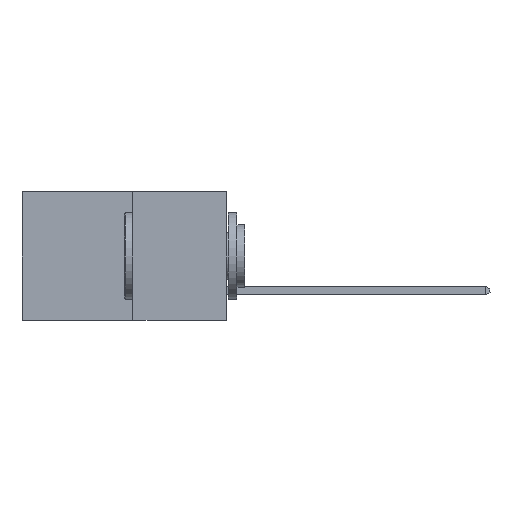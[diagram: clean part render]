
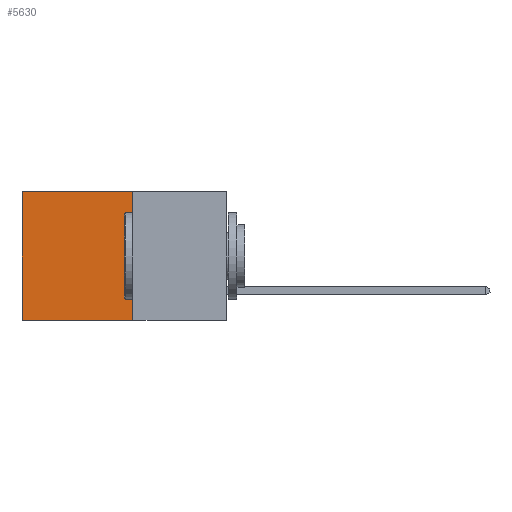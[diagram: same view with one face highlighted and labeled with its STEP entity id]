
A CAD part, left-side view. The second image highlights one B-rep face of the part: STEP entity #5630.
In plain terms, the highlighted planar face has unit normal (-1, 0, 0).
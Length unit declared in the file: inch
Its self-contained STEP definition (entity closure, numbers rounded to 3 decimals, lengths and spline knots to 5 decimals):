
#118 = VECTOR ( 'NONE', #5313, 39.37008 ) ;
#135 = DIRECTION ( 'NONE',  ( 0., 1., 0. ) ) ;
#157 = CARTESIAN_POINT ( 'NONE',  ( 0.277, 0.27, 0. ) ) ;
#957 = ORIENTED_EDGE ( 'NONE', *, *, #9601, .F. ) ;
#1545 = VERTEX_POINT ( 'NONE', #2370 ) ;
#1876 = VERTEX_POINT ( 'NONE', #6914 ) ;
#2260 = VECTOR ( 'NONE', #3214, 39.37008 ) ;
#2370 = CARTESIAN_POINT ( 'NONE',  ( 0.277, 0.59, -0.37 ) ) ;
#2439 = CARTESIAN_POINT ( 'NONE',  ( 0.277, 0.27, 0. ) ) ;
#2764 = ORIENTED_EDGE ( 'NONE', *, *, #3590, .T. ) ;
#3214 = DIRECTION ( 'NONE',  ( 0., 1., 0. ) ) ;
#3259 = VECTOR ( 'NONE', #135, 39.37008 ) ;
#3590 = EDGE_CURVE ( 'NONE', #1876, #1545, #8833, .T. ) ;
#3757 = LINE ( 'NONE', #5677, #7936 ) ;
#4158 = EDGE_LOOP ( 'NONE', ( #2764, #957, #7977, #9963 ) ) ;
#4512 = LINE ( 'NONE', #5747, #2260 ) ;
#4575 = FACE_OUTER_BOUND ( 'NONE', #4158, .T. ) ;
#5313 = DIRECTION ( 'NONE',  ( 0., 0., -1. ) ) ;
#5526 = LINE ( 'NONE', #2439, #3259 ) ;
#5547 = CARTESIAN_POINT ( 'NONE',  ( 0.277, 0.59, -0.37 ) ) ;
#5630 = ADVANCED_FACE ( 'NONE', ( #4575 ), #8061, .F. ) ;
#5632 = DIRECTION ( 'NONE',  ( 0., 0., -1. ) ) ;
#5677 = CARTESIAN_POINT ( 'NONE',  ( 0.277, 0.27, -0.37 ) ) ;
#5747 = CARTESIAN_POINT ( 'NONE',  ( 0.277, 0.27, -0.37 ) ) ;
#6056 = VERTEX_POINT ( 'NONE', #6475 ) ;
#6214 = EDGE_CURVE ( 'NONE', #8110, #6056, #3757, .T. ) ;
#6475 = CARTESIAN_POINT ( 'NONE',  ( 0.277, 0.27, -0.37 ) ) ;
#6914 = CARTESIAN_POINT ( 'NONE',  ( 0.277, 0.59, 0. ) ) ;
#7552 = DIRECTION ( 'NONE',  ( 0., 0., -1. ) ) ;
#7564 = DIRECTION ( 'NONE',  ( 1., 0., 0. ) ) ;
#7693 = EDGE_CURVE ( 'NONE', #8110, #1876, #5526, .T. ) ;
#7936 = VECTOR ( 'NONE', #5632, 39.37008 ) ;
#7977 = ORIENTED_EDGE ( 'NONE', *, *, #6214, .F. ) ;
#8061 = PLANE ( 'NONE',  #8114 ) ;
#8110 = VERTEX_POINT ( 'NONE', #157 ) ;
#8114 = AXIS2_PLACEMENT_3D ( 'NONE', #8123, #7564, #7552 ) ;
#8123 = CARTESIAN_POINT ( 'NONE',  ( 0.277, 0.27, -0.37 ) ) ;
#8833 = LINE ( 'NONE', #5547, #118 ) ;
#9601 = EDGE_CURVE ( 'NONE', #6056, #1545, #4512, .T. ) ;
#9963 = ORIENTED_EDGE ( 'NONE', *, *, #7693, .T. ) ;
